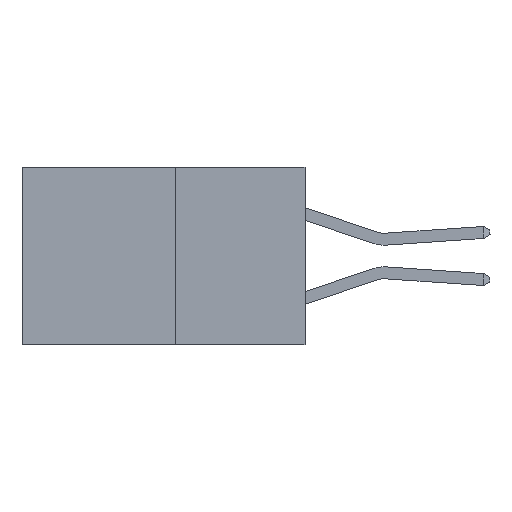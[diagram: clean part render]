
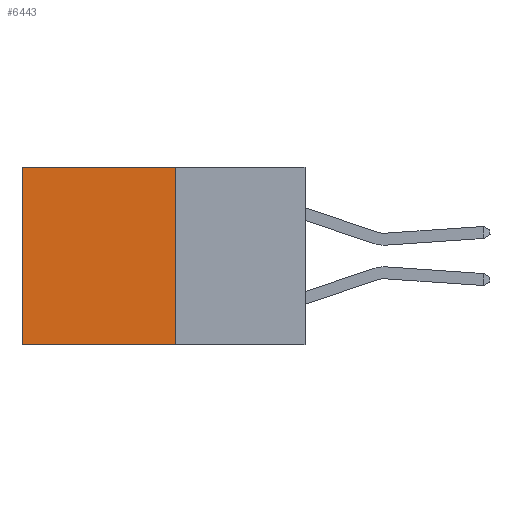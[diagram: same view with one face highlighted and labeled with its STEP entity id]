
A CAD part, left-side view. The second image highlights one B-rep face of the part: STEP entity #6443.
In plain terms, the highlighted planar face has unit normal (-1, 0, 0).
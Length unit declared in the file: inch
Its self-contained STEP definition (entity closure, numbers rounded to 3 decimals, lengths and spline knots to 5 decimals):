
#390 = CARTESIAN_POINT ( 'NONE',  ( 0.277, 0.59, 0. ) ) ;
#957 = LINE ( 'NONE', #1613, #13835 ) ;
#1613 = CARTESIAN_POINT ( 'NONE',  ( 0.277, 0.27, 0. ) ) ;
#2443 = LINE ( 'NONE', #3332, #29828 ) ;
#2475 = LINE ( 'NONE', #15537, #16234 ) ;
#3332 = CARTESIAN_POINT ( 'NONE',  ( 0.277, 0.27, -0.37 ) ) ;
#3799 = CARTESIAN_POINT ( 'NONE',  ( 0.277, 0.27, -0.37 ) ) ;
#3940 = AXIS2_PLACEMENT_3D ( 'NONE', #3799, #22952, #6594 ) ;
#4650 = EDGE_CURVE ( 'NONE', #22713, #14510, #2475, .T. ) ;
#5721 = DIRECTION ( 'NONE',  ( 0., 0., -1. ) ) ;
#6443 = ADVANCED_FACE ( 'NONE', ( #15269 ), #30539, .F. ) ;
#6594 = DIRECTION ( 'NONE',  ( 0., 0., -1. ) ) ;
#6638 = ORIENTED_EDGE ( 'NONE', *, *, #16156, .T. ) ;
#10181 = DIRECTION ( 'NONE',  ( 0., 0., -1. ) ) ;
#13209 = EDGE_CURVE ( 'NONE', #14510, #26547, #2443, .T. ) ;
#13835 = VECTOR ( 'NONE', #26287, 39.37008 ) ;
#14510 = VERTEX_POINT ( 'NONE', #30502 ) ;
#14960 = CARTESIAN_POINT ( 'NONE',  ( 0.277, 0.27, 0. ) ) ;
#15269 = FACE_OUTER_BOUND ( 'NONE', #25118, .T. ) ;
#15537 = CARTESIAN_POINT ( 'NONE',  ( 0.277, 0.27, -0.37 ) ) ;
#16156 = EDGE_CURVE ( 'NONE', #22713, #26483, #957, .T. ) ;
#16234 = VECTOR ( 'NONE', #10181, 39.37008 ) ;
#17951 = ORIENTED_EDGE ( 'NONE', *, *, #19413, .T. ) ;
#19270 = ORIENTED_EDGE ( 'NONE', *, *, #4650, .F. ) ;
#19413 = EDGE_CURVE ( 'NONE', #26483, #26547, #27031, .T. ) ;
#22713 = VERTEX_POINT ( 'NONE', #14960 ) ;
#22952 = DIRECTION ( 'NONE',  ( 1., 0., 0. ) ) ;
#24845 = CARTESIAN_POINT ( 'NONE',  ( 0.277, 0.59, -0.37 ) ) ;
#25118 = EDGE_LOOP ( 'NONE', ( #17951, #27362, #19270, #6638 ) ) ;
#26287 = DIRECTION ( 'NONE',  ( 0., 1., 0. ) ) ;
#26483 = VERTEX_POINT ( 'NONE', #390 ) ;
#26547 = VERTEX_POINT ( 'NONE', #30662 ) ;
#27031 = LINE ( 'NONE', #24845, #35119 ) ;
#27362 = ORIENTED_EDGE ( 'NONE', *, *, #13209, .F. ) ;
#27998 = DIRECTION ( 'NONE',  ( 0., 1., 0. ) ) ;
#29828 = VECTOR ( 'NONE', #27998, 39.37008 ) ;
#30502 = CARTESIAN_POINT ( 'NONE',  ( 0.277, 0.27, -0.37 ) ) ;
#30539 = PLANE ( 'NONE',  #3940 ) ;
#30662 = CARTESIAN_POINT ( 'NONE',  ( 0.277, 0.59, -0.37 ) ) ;
#35119 = VECTOR ( 'NONE', #5721, 39.37008 ) ;
